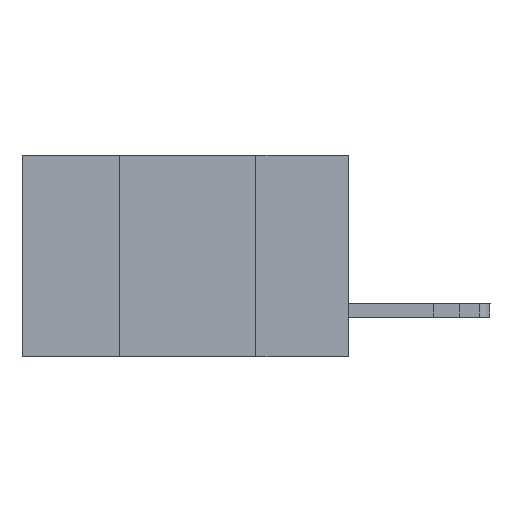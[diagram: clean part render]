
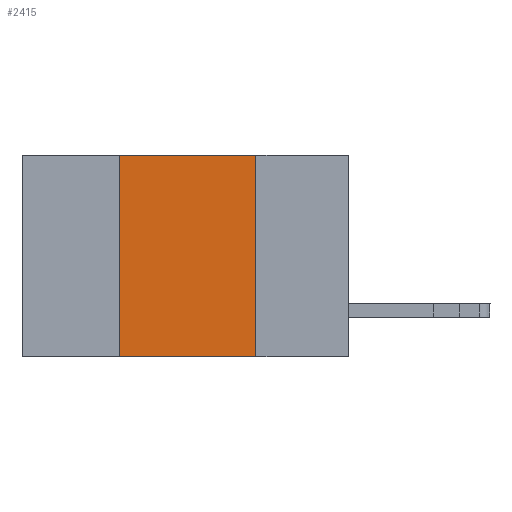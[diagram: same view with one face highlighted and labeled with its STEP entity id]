
A CAD part, left-side view. The second image highlights one B-rep face of the part: STEP entity #2415.
In plain terms, the highlighted planar face has unit normal (-1, 0, 0).
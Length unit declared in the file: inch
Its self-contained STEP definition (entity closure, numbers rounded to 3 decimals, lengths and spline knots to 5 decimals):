
#122 = DIRECTION ( 'NONE',  ( 1., 0., 0. ) ) ;
#395 = VERTEX_POINT ( 'NONE', #955 ) ;
#498 = VECTOR ( 'NONE', #7942, 39.37008 ) ;
#754 = PLANE ( 'NONE',  #10186 ) ;
#849 = EDGE_CURVE ( 'NONE', #8549, #6806, #2450, .T. ) ;
#955 = CARTESIAN_POINT ( 'NONE',  ( 0., 0.17, -0.37 ) ) ;
#1592 = DIRECTION ( 'NONE',  ( 0., 0., -1. ) ) ;
#1664 = LINE ( 'NONE', #9618, #5243 ) ;
#1831 = DIRECTION ( 'NONE',  ( 0., 0., 1. ) ) ;
#2415 = ADVANCED_FACE ( 'NONE', ( #4108 ), #754, .F. ) ;
#2445 = DIRECTION ( 'NONE',  ( 0., -1., 0. ) ) ;
#2447 = DIRECTION ( 'NONE',  ( 0., 0., -1. ) ) ;
#2450 = LINE ( 'NONE', #7166, #498 ) ;
#3062 = CARTESIAN_POINT ( 'NONE',  ( 0., 0.42, 0. ) ) ;
#3290 = EDGE_CURVE ( 'NONE', #6806, #395, #8776, .T. ) ;
#3647 = EDGE_LOOP ( 'NONE', ( #5852, #5893, #8344, #7595 ) ) ;
#4108 = FACE_OUTER_BOUND ( 'NONE', #3647, .T. ) ;
#4594 = VECTOR ( 'NONE', #2447, 39.37008 ) ;
#5243 = VECTOR ( 'NONE', #2445, 39.37008 ) ;
#5586 = CARTESIAN_POINT ( 'NONE',  ( 0., 0.6, 0. ) ) ;
#5786 = LINE ( 'NONE', #8887, #9429 ) ;
#5852 = ORIENTED_EDGE ( 'NONE', *, *, #3290, .F. ) ;
#5893 = ORIENTED_EDGE ( 'NONE', *, *, #849, .F. ) ;
#6806 = VERTEX_POINT ( 'NONE', #7829 ) ;
#7166 = CARTESIAN_POINT ( 'NONE',  ( 0., 0.6, 0. ) ) ;
#7216 = CARTESIAN_POINT ( 'NONE',  ( 0., 0.17, -0.37 ) ) ;
#7595 = ORIENTED_EDGE ( 'NONE', *, *, #8281, .T. ) ;
#7829 = CARTESIAN_POINT ( 'NONE',  ( 0., 0.17, 0. ) ) ;
#7942 = DIRECTION ( 'NONE',  ( 0., -1., 0. ) ) ;
#8281 = EDGE_CURVE ( 'NONE', #8663, #395, #1664, .T. ) ;
#8344 = ORIENTED_EDGE ( 'NONE', *, *, #9601, .F. ) ;
#8549 = VERTEX_POINT ( 'NONE', #3062 ) ;
#8663 = VERTEX_POINT ( 'NONE', #8957 ) ;
#8776 = LINE ( 'NONE', #7216, #4594 ) ;
#8887 = CARTESIAN_POINT ( 'NONE',  ( 0., 0.42, -0.37 ) ) ;
#8957 = CARTESIAN_POINT ( 'NONE',  ( 0., 0.42, -0.37 ) ) ;
#9429 = VECTOR ( 'NONE', #1831, 39.37008 ) ;
#9601 = EDGE_CURVE ( 'NONE', #8663, #8549, #5786, .T. ) ;
#9618 = CARTESIAN_POINT ( 'NONE',  ( 0., 0.6, -0.37 ) ) ;
#10186 = AXIS2_PLACEMENT_3D ( 'NONE', #5586, #122, #1592 ) ;
